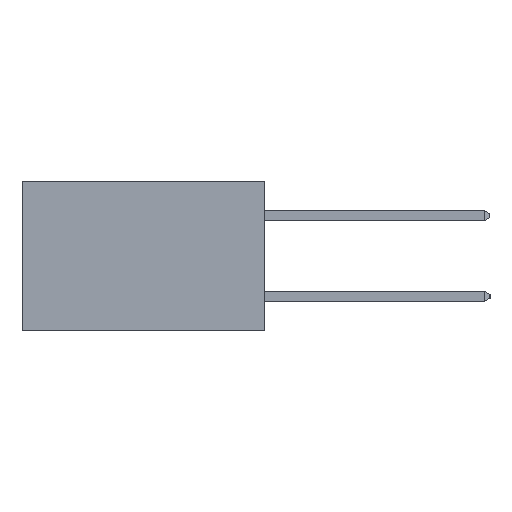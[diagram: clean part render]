
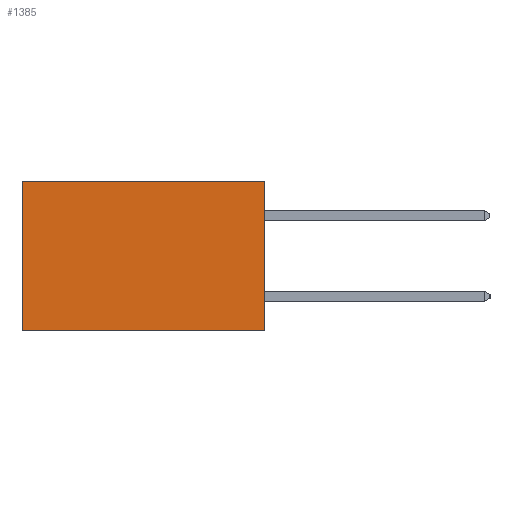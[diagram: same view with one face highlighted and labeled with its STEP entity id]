
A CAD part, left-side view. The second image highlights one B-rep face of the part: STEP entity #1385.
In plain terms, the highlighted planar face has unit normal (-1, 0, 0).
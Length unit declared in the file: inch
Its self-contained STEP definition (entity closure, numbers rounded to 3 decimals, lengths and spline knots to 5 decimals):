
#32 = VERTEX_POINT ( 'NONE', #783 ) ;
#444 = EDGE_CURVE ( 'NONE', #8617, #32, #11724, .T. ) ;
#527 = EDGE_CURVE ( 'NONE', #7509, #8617, #8795, .T. ) ;
#783 = CARTESIAN_POINT ( 'NONE',  ( 0.2615, 0.6, -0.37 ) ) ;
#887 = PLANE ( 'NONE',  #1953 ) ;
#1385 = ADVANCED_FACE ( 'NONE', ( #13625 ), #887, .F. ) ;
#1953 = AXIS2_PLACEMENT_3D ( 'NONE', #13878, #13854, #13837 ) ;
#2642 = EDGE_CURVE ( 'NONE', #11589, #32, #11617, .T. ) ;
#2662 = ORIENTED_EDGE ( 'NONE', *, *, #444, .F. ) ;
#2789 = CARTESIAN_POINT ( 'NONE',  ( 0.2615, 0., -0.37 ) ) ;
#3145 = VECTOR ( 'NONE', #5418, 39.37008 ) ;
#3908 = DIRECTION ( 'NONE',  ( 0., 0., -1. ) ) ;
#4085 = CARTESIAN_POINT ( 'NONE',  ( 0.2615, 0.6, -0.37 ) ) ;
#4266 = CARTESIAN_POINT ( 'NONE',  ( 0.2615, 0.6, 0. ) ) ;
#5397 = EDGE_LOOP ( 'NONE', ( #10783, #2662, #5522, #11109 ) ) ;
#5418 = DIRECTION ( 'NONE',  ( 0., 0., -1. ) ) ;
#5522 = ORIENTED_EDGE ( 'NONE', *, *, #527, .F. ) ;
#5794 = CARTESIAN_POINT ( 'NONE',  ( 0.2615, 0., -0.37 ) ) ;
#6569 = CARTESIAN_POINT ( 'NONE',  ( 0.2615, 0., 0. ) ) ;
#7013 = EDGE_CURVE ( 'NONE', #7509, #11589, #10901, .T. ) ;
#7385 = VECTOR ( 'NONE', #13433, 39.37008 ) ;
#7509 = VERTEX_POINT ( 'NONE', #6569 ) ;
#8617 = VERTEX_POINT ( 'NONE', #5794 ) ;
#8795 = LINE ( 'NONE', #9133, #3145 ) ;
#8852 = VECTOR ( 'NONE', #3908, 39.37008 ) ;
#9133 = CARTESIAN_POINT ( 'NONE',  ( 0.2615, 0., -0.37 ) ) ;
#10209 = VECTOR ( 'NONE', #11331, 39.37008 ) ;
#10783 = ORIENTED_EDGE ( 'NONE', *, *, #2642, .T. ) ;
#10901 = LINE ( 'NONE', #13649, #10209 ) ;
#11109 = ORIENTED_EDGE ( 'NONE', *, *, #7013, .T. ) ;
#11331 = DIRECTION ( 'NONE',  ( 0., 1., 0. ) ) ;
#11589 = VERTEX_POINT ( 'NONE', #4266 ) ;
#11617 = LINE ( 'NONE', #4085, #8852 ) ;
#11724 = LINE ( 'NONE', #2789, #7385 ) ;
#13433 = DIRECTION ( 'NONE',  ( 0., 1., 0. ) ) ;
#13625 = FACE_OUTER_BOUND ( 'NONE', #5397, .T. ) ;
#13649 = CARTESIAN_POINT ( 'NONE',  ( 0.2615, 0., 0. ) ) ;
#13837 = DIRECTION ( 'NONE',  ( 0., 0., -1. ) ) ;
#13854 = DIRECTION ( 'NONE',  ( 1., 0., 0. ) ) ;
#13878 = CARTESIAN_POINT ( 'NONE',  ( 0.2615, 0., -0.37 ) ) ;
